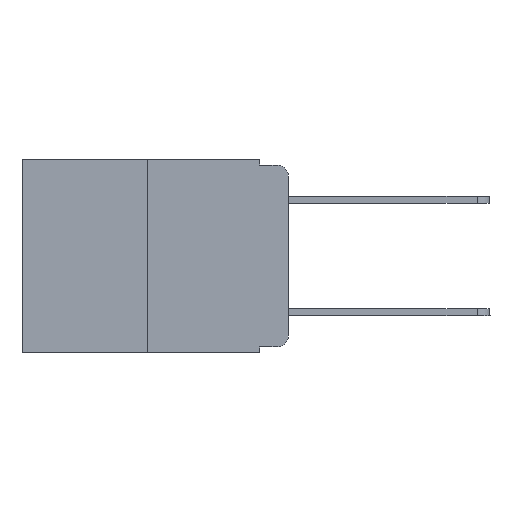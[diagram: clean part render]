
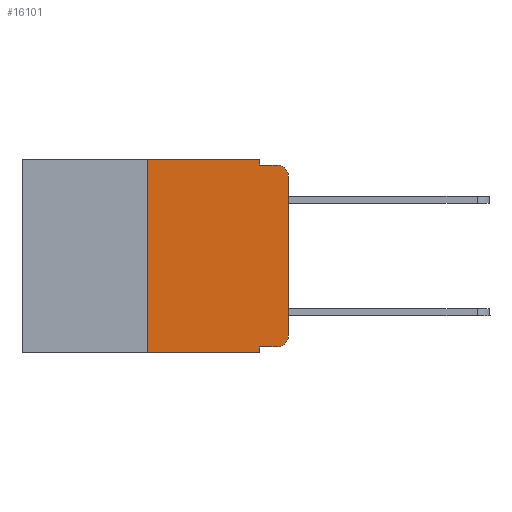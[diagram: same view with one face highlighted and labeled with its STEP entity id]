
A CAD part, left-side view. The second image highlights one B-rep face of the part: STEP entity #16101.
In plain terms, the highlighted planar face has unit normal (-1, 0, 0).
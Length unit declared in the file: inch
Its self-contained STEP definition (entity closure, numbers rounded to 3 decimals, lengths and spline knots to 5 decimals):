
#478 = LINE ( 'NONE', #7007, #19306 ) ;
#814 = EDGE_CURVE ( 'NONE', #6271, #13186, #20071, .T. ) ;
#952 = CARTESIAN_POINT ( 'NONE',  ( 0., 0.25, 0. ) ) ;
#1082 = DIRECTION ( 'NONE',  ( 0., 0., -1. ) ) ;
#1222 = CARTESIAN_POINT ( 'NONE',  ( 0., 0.051, 0. ) ) ;
#1724 = ORIENTED_EDGE ( 'NONE', *, *, #13371, .F. ) ;
#1988 = AXIS2_PLACEMENT_3D ( 'NONE', #17436, #15791, #1082 ) ;
#2152 = EDGE_CURVE ( 'NONE', #3981, #20434, #478, .T. ) ;
#2325 = VERTEX_POINT ( 'NONE', #6178 ) ;
#2362 = CIRCLE ( 'NONE', #20554, 0.02 ) ;
#2922 = ORIENTED_EDGE ( 'NONE', *, *, #17045, .T. ) ;
#3703 = VECTOR ( 'NONE', #15556, 39.37008 ) ;
#3729 = CARTESIAN_POINT ( 'NONE',  ( 0., 0.051, 0. ) ) ;
#3911 = CARTESIAN_POINT ( 'NONE',  ( 0., 0.02, -0.03 ) ) ;
#3981 = VERTEX_POINT ( 'NONE', #4277 ) ;
#4011 = CARTESIAN_POINT ( 'NONE',  ( 0., 0.25, -0.343 ) ) ;
#4054 = EDGE_LOOP ( 'NONE', ( #18585, #17647, #1724, #18659, #5624, #12863, #2922, #20095, #12624, #8886 ) ) ;
#4240 = LINE ( 'NONE', #1222, #20320 ) ;
#4277 = CARTESIAN_POINT ( 'NONE',  ( 0., 0., -0.313 ) ) ;
#4450 = VECTOR ( 'NONE', #20791, 39.37008 ) ;
#4451 = CIRCLE ( 'NONE', #16424, 0.02 ) ;
#4810 = LINE ( 'NONE', #11399, #16019 ) ;
#4894 = DIRECTION ( 'NONE',  ( 0., -1., 0. ) ) ;
#5207 = LINE ( 'NONE', #19736, #7440 ) ;
#5624 = ORIENTED_EDGE ( 'NONE', *, *, #15869, .F. ) ;
#6178 = CARTESIAN_POINT ( 'NONE',  ( 0., 0.051, -0.343 ) ) ;
#6271 = VERTEX_POINT ( 'NONE', #19740 ) ;
#6749 = VECTOR ( 'NONE', #18719, 39.37008 ) ;
#6904 = VERTEX_POINT ( 'NONE', #11948 ) ;
#7007 = CARTESIAN_POINT ( 'NONE',  ( 0., 0., 0. ) ) ;
#7440 = VECTOR ( 'NONE', #4894, 39.37008 ) ;
#7493 = VECTOR ( 'NONE', #13572, 39.37008 ) ;
#7505 = CARTESIAN_POINT ( 'NONE',  ( 0., 0.051, -0.01 ) ) ;
#7773 = EDGE_CURVE ( 'NONE', #10876, #20443, #9004, .T. ) ;
#8886 = ORIENTED_EDGE ( 'NONE', *, *, #16639, .T. ) ;
#9004 = LINE ( 'NONE', #952, #3703 ) ;
#9570 = EDGE_CURVE ( 'NONE', #20434, #6904, #4451, .T. ) ;
#9772 = DIRECTION ( 'NONE',  ( 0., -1., 0. ) ) ;
#10473 = DIRECTION ( 'NONE',  ( -1., 0., 0. ) ) ;
#10856 = DIRECTION ( 'NONE',  ( -1., 0., 0. ) ) ;
#10876 = VERTEX_POINT ( 'NONE', #4011 ) ;
#10889 = FACE_OUTER_BOUND ( 'NONE', #4054, .T. ) ;
#10938 = CARTESIAN_POINT ( 'NONE',  ( 0., 0.473, -0.343 ) ) ;
#11399 = CARTESIAN_POINT ( 'NONE',  ( 0., 0.051, -0.01 ) ) ;
#11770 = VERTEX_POINT ( 'NONE', #14065 ) ;
#11948 = CARTESIAN_POINT ( 'NONE',  ( 0., 0.02, -0.01 ) ) ;
#12235 = VERTEX_POINT ( 'NONE', #19959 ) ;
#12624 = ORIENTED_EDGE ( 'NONE', *, *, #12628, .T. ) ;
#12628 = EDGE_CURVE ( 'NONE', #11770, #12235, #5207, .T. ) ;
#12863 = ORIENTED_EDGE ( 'NONE', *, *, #7773, .F. ) ;
#13186 = VERTEX_POINT ( 'NONE', #7505 ) ;
#13371 = EDGE_CURVE ( 'NONE', #13186, #6904, #4810, .T. ) ;
#13466 = LINE ( 'NONE', #20108, #7493 ) ;
#13572 = DIRECTION ( 'NONE',  ( 0., -1., 0. ) ) ;
#13976 = CARTESIAN_POINT ( 'NONE',  ( 0., 0., -0.03 ) ) ;
#14065 = CARTESIAN_POINT ( 'NONE',  ( 0., 0.051, -0.333 ) ) ;
#14362 = LINE ( 'NONE', #10938, #4450 ) ;
#14383 = CARTESIAN_POINT ( 'NONE',  ( 0., 0.02, -0.313 ) ) ;
#15556 = DIRECTION ( 'NONE',  ( 0., 0., 1. ) ) ;
#15791 = DIRECTION ( 'NONE',  ( 1., 0., 0. ) ) ;
#15869 = EDGE_CURVE ( 'NONE', #20443, #6271, #13466, .T. ) ;
#16019 = VECTOR ( 'NONE', #9772, 39.37008 ) ;
#16070 = DIRECTION ( 'NONE',  ( 0., 0., -1. ) ) ;
#16101 = ADVANCED_FACE ( 'NONE', ( #10889 ), #20427, .F. ) ;
#16424 = AXIS2_PLACEMENT_3D ( 'NONE', #3911, #10473, #17026 ) ;
#16639 = EDGE_CURVE ( 'NONE', #12235, #3981, #2362, .T. ) ;
#16929 = DIRECTION ( 'NONE',  ( 0., 0., 1. ) ) ;
#17026 = DIRECTION ( 'NONE',  ( 0., 0., -1. ) ) ;
#17045 = EDGE_CURVE ( 'NONE', #10876, #2325, #14362, .T. ) ;
#17314 = CARTESIAN_POINT ( 'NONE',  ( 0., 0.25, 0. ) ) ;
#17436 = CARTESIAN_POINT ( 'NONE',  ( 0., 0.473, 0. ) ) ;
#17647 = ORIENTED_EDGE ( 'NONE', *, *, #9570, .T. ) ;
#18585 = ORIENTED_EDGE ( 'NONE', *, *, #2152, .T. ) ;
#18659 = ORIENTED_EDGE ( 'NONE', *, *, #814, .F. ) ;
#18719 = DIRECTION ( 'NONE',  ( 0., 0., -1. ) ) ;
#18984 = DIRECTION ( 'NONE',  ( 0., 0., -1. ) ) ;
#19306 = VECTOR ( 'NONE', #16929, 39.37008 ) ;
#19736 = CARTESIAN_POINT ( 'NONE',  ( 0., 0.051, -0.333 ) ) ;
#19740 = CARTESIAN_POINT ( 'NONE',  ( 0., 0.051, 0. ) ) ;
#19959 = CARTESIAN_POINT ( 'NONE',  ( 0., 0.02, -0.333 ) ) ;
#20071 = LINE ( 'NONE', #3729, #6749 ) ;
#20095 = ORIENTED_EDGE ( 'NONE', *, *, #20878, .F. ) ;
#20108 = CARTESIAN_POINT ( 'NONE',  ( 0., 0.473, 0. ) ) ;
#20320 = VECTOR ( 'NONE', #18984, 39.37008 ) ;
#20427 = PLANE ( 'NONE',  #1988 ) ;
#20434 = VERTEX_POINT ( 'NONE', #13976 ) ;
#20443 = VERTEX_POINT ( 'NONE', #17314 ) ;
#20554 = AXIS2_PLACEMENT_3D ( 'NONE', #14383, #10856, #16070 ) ;
#20791 = DIRECTION ( 'NONE',  ( 0., -1., 0. ) ) ;
#20878 = EDGE_CURVE ( 'NONE', #11770, #2325, #4240, .T. ) ;
